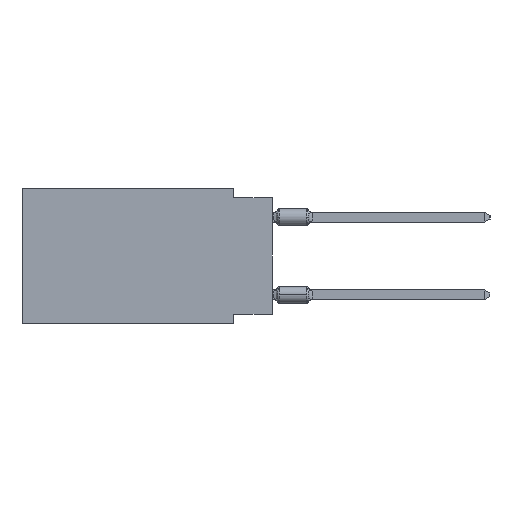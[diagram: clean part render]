
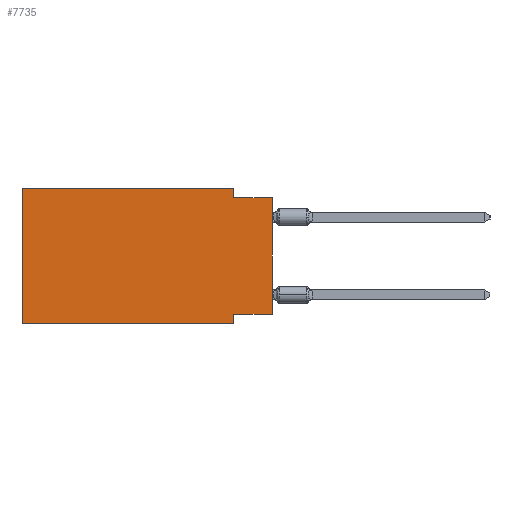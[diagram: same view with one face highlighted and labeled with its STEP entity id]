
A CAD part, left-side view. The second image highlights one B-rep face of the part: STEP entity #7735.
In plain terms, the highlighted planar face has unit normal (-1, 0, 0).
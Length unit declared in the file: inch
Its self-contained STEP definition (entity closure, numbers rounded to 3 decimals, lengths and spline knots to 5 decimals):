
#384 = DIRECTION ( 'NONE',  ( 0., -1., 0. ) ) ;
#701 = VERTEX_POINT ( 'NONE', #35774 ) ;
#1432 = DIRECTION ( 'NONE',  ( 1., 0., 0. ) ) ;
#1659 = EDGE_CURVE ( 'NONE', #43254, #41492, #13003, .T. ) ;
#1682 = CARTESIAN_POINT ( 'NONE',  ( 0., 0.1, -0.35 ) ) ;
#1968 = FACE_OUTER_BOUND ( 'NONE', #41671, .T. ) ;
#4298 = VECTOR ( 'NONE', #41472, 39.37008 ) ;
#4695 = EDGE_CURVE ( 'NONE', #28275, #4857, #10439, .T. ) ;
#4857 = VERTEX_POINT ( 'NONE', #44273 ) ;
#5328 = LINE ( 'NONE', #45878, #6074 ) ;
#5331 = VERTEX_POINT ( 'NONE', #1682 ) ;
#5639 = DIRECTION ( 'NONE',  ( 0., 1., 0. ) ) ;
#5955 = DIRECTION ( 'NONE',  ( 0., 0., 1. ) ) ;
#6074 = VECTOR ( 'NONE', #46419, 39.37008 ) ;
#6509 = DIRECTION ( 'NONE',  ( 0., 0., -1. ) ) ;
#7735 = ADVANCED_FACE ( 'NONE', ( #1968 ), #22904, .F. ) ;
#7873 = CARTESIAN_POINT ( 'NONE',  ( 0., 0.1, 0. ) ) ;
#8609 = VERTEX_POINT ( 'NONE', #41451 ) ;
#8708 = DIRECTION ( 'NONE',  ( 0., 0., -1. ) ) ;
#9020 = DIRECTION ( 'NONE',  ( 0., 0., -1. ) ) ;
#10078 = LINE ( 'NONE', #38584, #18718 ) ;
#10439 = LINE ( 'NONE', #22027, #46080 ) ;
#11580 = EDGE_CURVE ( 'NONE', #701, #12530, #5328, .T. ) ;
#12530 = VERTEX_POINT ( 'NONE', #7873 ) ;
#12731 = LINE ( 'NONE', #21061, #4298 ) ;
#13003 = LINE ( 'NONE', #50348, #28205 ) ;
#17273 = ORIENTED_EDGE ( 'NONE', *, *, #37880, .F. ) ;
#17603 = ORIENTED_EDGE ( 'NONE', *, *, #4695, .F. ) ;
#18718 = VECTOR ( 'NONE', #37793, 39.37008 ) ;
#18954 = VECTOR ( 'NONE', #9020, 39.37008 ) ;
#21061 = CARTESIAN_POINT ( 'NONE',  ( 0., 0.645, 0. ) ) ;
#21193 = VECTOR ( 'NONE', #5955, 39.37008 ) ;
#22027 = CARTESIAN_POINT ( 'NONE',  ( 0., 0., -0.325 ) ) ;
#22904 = PLANE ( 'NONE',  #34230 ) ;
#25286 = CARTESIAN_POINT ( 'NONE',  ( 0., 0., -0.025 ) ) ;
#25981 = EDGE_CURVE ( 'NONE', #8609, #5331, #10078, .T. ) ;
#26379 = LINE ( 'NONE', #38466, #21193 ) ;
#27256 = ORIENTED_EDGE ( 'NONE', *, *, #47063, .T. ) ;
#28205 = VECTOR ( 'NONE', #384, 39.37008 ) ;
#28275 = VERTEX_POINT ( 'NONE', #41331 ) ;
#28533 = ORIENTED_EDGE ( 'NONE', *, *, #25981, .T. ) ;
#28859 = EDGE_CURVE ( 'NONE', #4857, #5331, #33992, .T. ) ;
#29122 = LINE ( 'NONE', #45510, #32587 ) ;
#29803 = ORIENTED_EDGE ( 'NONE', *, *, #11580, .F. ) ;
#32587 = VECTOR ( 'NONE', #8708, 39.37008 ) ;
#33992 = LINE ( 'NONE', #42327, #18954 ) ;
#34230 = AXIS2_PLACEMENT_3D ( 'NONE', #46817, #1432, #6509 ) ;
#35774 = CARTESIAN_POINT ( 'NONE',  ( 0., 0.645, 0. ) ) ;
#37793 = DIRECTION ( 'NONE',  ( 0., -1., 0. ) ) ;
#37880 = EDGE_CURVE ( 'NONE', #12530, #43254, #29122, .T. ) ;
#37885 = EDGE_CURVE ( 'NONE', #8609, #701, #12731, .T. ) ;
#38466 = CARTESIAN_POINT ( 'NONE',  ( 0., 0., 0. ) ) ;
#38584 = CARTESIAN_POINT ( 'NONE',  ( 0., 0.645, -0.35 ) ) ;
#41331 = CARTESIAN_POINT ( 'NONE',  ( 0., 0., -0.325 ) ) ;
#41451 = CARTESIAN_POINT ( 'NONE',  ( 0., 0.645, -0.35 ) ) ;
#41472 = DIRECTION ( 'NONE',  ( 0., 0., 1. ) ) ;
#41492 = VERTEX_POINT ( 'NONE', #25286 ) ;
#41671 = EDGE_LOOP ( 'NONE', ( #27256, #50479, #17273, #29803, #43033, #28533, #48080, #17603 ) ) ;
#42327 = CARTESIAN_POINT ( 'NONE',  ( 0., 0.1, -0.35 ) ) ;
#43033 = ORIENTED_EDGE ( 'NONE', *, *, #37885, .F. ) ;
#43254 = VERTEX_POINT ( 'NONE', #50743 ) ;
#44273 = CARTESIAN_POINT ( 'NONE',  ( 0., 0.1, -0.325 ) ) ;
#45510 = CARTESIAN_POINT ( 'NONE',  ( 0., 0.1, 0. ) ) ;
#45878 = CARTESIAN_POINT ( 'NONE',  ( 0., 0.645, 0. ) ) ;
#46080 = VECTOR ( 'NONE', #5639, 39.37008 ) ;
#46419 = DIRECTION ( 'NONE',  ( 0., -1., 0. ) ) ;
#46817 = CARTESIAN_POINT ( 'NONE',  ( 0., 0.645, 0. ) ) ;
#47063 = EDGE_CURVE ( 'NONE', #28275, #41492, #26379, .T. ) ;
#48080 = ORIENTED_EDGE ( 'NONE', *, *, #28859, .F. ) ;
#50348 = CARTESIAN_POINT ( 'NONE',  ( 0., 0., -0.025 ) ) ;
#50479 = ORIENTED_EDGE ( 'NONE', *, *, #1659, .F. ) ;
#50743 = CARTESIAN_POINT ( 'NONE',  ( 0., 0.1, -0.025 ) ) ;
